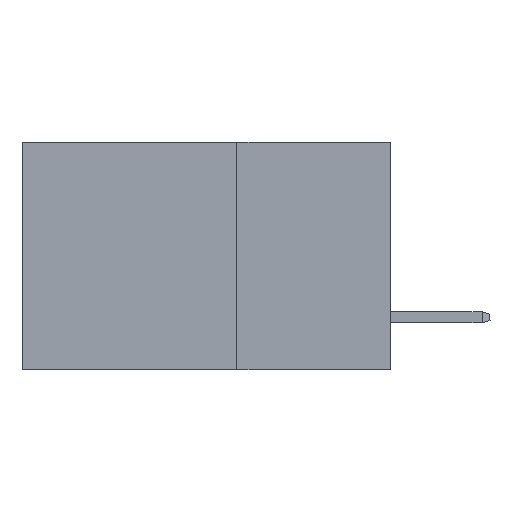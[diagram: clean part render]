
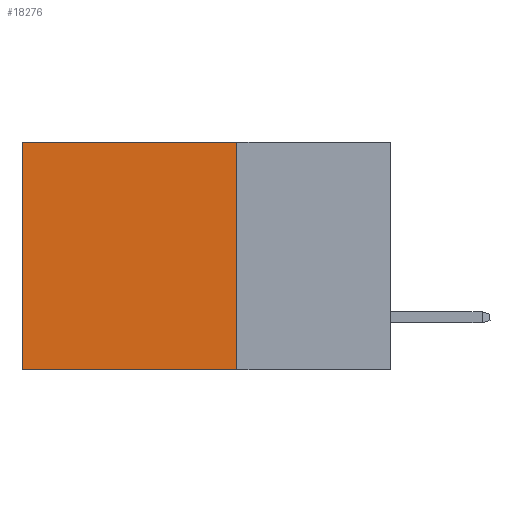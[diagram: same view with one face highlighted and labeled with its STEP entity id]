
A CAD part, left-side view. The second image highlights one B-rep face of the part: STEP entity #18276.
In plain terms, the highlighted planar face has unit normal (-1, 0, 0).
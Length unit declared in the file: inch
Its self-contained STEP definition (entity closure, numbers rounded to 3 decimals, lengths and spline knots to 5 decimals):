
#1035 = PLANE ( 'NONE',  #15582 ) ;
#1772 = VERTEX_POINT ( 'NONE', #13681 ) ;
#2422 = VECTOR ( 'NONE', #20571, 39.37008 ) ;
#3056 = CARTESIAN_POINT ( 'NONE',  ( 0.2875, 0.25, 0. ) ) ;
#3220 = VECTOR ( 'NONE', #11696, 39.37008 ) ;
#3311 = ORIENTED_EDGE ( 'NONE', *, *, #23313, .T. ) ;
#3791 = CARTESIAN_POINT ( 'NONE',  ( 0.2875, 0.25, 0. ) ) ;
#4580 = ORIENTED_EDGE ( 'NONE', *, *, #14862, .F. ) ;
#5068 = DIRECTION ( 'NONE',  ( 1., 0., 0. ) ) ;
#5829 = DIRECTION ( 'NONE',  ( 0., 0., -1. ) ) ;
#6169 = VERTEX_POINT ( 'NONE', #10185 ) ;
#6602 = CARTESIAN_POINT ( 'NONE',  ( 0.2875, 0.25, 0. ) ) ;
#7557 = VECTOR ( 'NONE', #5829, 39.37008 ) ;
#7774 = LINE ( 'NONE', #12406, #2422 ) ;
#10185 = CARTESIAN_POINT ( 'NONE',  ( 0.2875, 0.6, -0.37 ) ) ;
#11323 = ORIENTED_EDGE ( 'NONE', *, *, #19201, .F. ) ;
#11696 = DIRECTION ( 'NONE',  ( 0., 0., -1. ) ) ;
#11820 = LINE ( 'NONE', #6602, #21333 ) ;
#12406 = CARTESIAN_POINT ( 'NONE',  ( 0.2875, 0.25, -0.37 ) ) ;
#13412 = VERTEX_POINT ( 'NONE', #14304 ) ;
#13681 = CARTESIAN_POINT ( 'NONE',  ( 0.2875, 0.6, 0. ) ) ;
#14304 = CARTESIAN_POINT ( 'NONE',  ( 0.2875, 0.25, -0.37 ) ) ;
#14862 = EDGE_CURVE ( 'NONE', #13412, #6169, #7774, .T. ) ;
#15582 = AXIS2_PLACEMENT_3D ( 'NONE', #3056, #5068, #19332 ) ;
#16898 = DIRECTION ( 'NONE',  ( 0., 1., 0. ) ) ;
#18276 = ADVANCED_FACE ( 'NONE', ( #21880 ), #1035, .F. ) ;
#19201 = EDGE_CURVE ( 'NONE', #22407, #13412, #23666, .T. ) ;
#19332 = DIRECTION ( 'NONE',  ( 0., 0., -1. ) ) ;
#19904 = EDGE_LOOP ( 'NONE', ( #3311, #4580, #11323, #23877 ) ) ;
#20571 = DIRECTION ( 'NONE',  ( 0., 1., 0. ) ) ;
#21333 = VECTOR ( 'NONE', #16898, 39.37008 ) ;
#21880 = FACE_OUTER_BOUND ( 'NONE', #19904, .T. ) ;
#22362 = EDGE_CURVE ( 'NONE', #22407, #1772, #11820, .T. ) ;
#22407 = VERTEX_POINT ( 'NONE', #24933 ) ;
#23313 = EDGE_CURVE ( 'NONE', #1772, #6169, #24044, .T. ) ;
#23666 = LINE ( 'NONE', #3791, #7557 ) ;
#23769 = CARTESIAN_POINT ( 'NONE',  ( 0.2875, 0.6, 0. ) ) ;
#23877 = ORIENTED_EDGE ( 'NONE', *, *, #22362, .T. ) ;
#24044 = LINE ( 'NONE', #23769, #3220 ) ;
#24933 = CARTESIAN_POINT ( 'NONE',  ( 0.2875, 0.25, 0. ) ) ;
